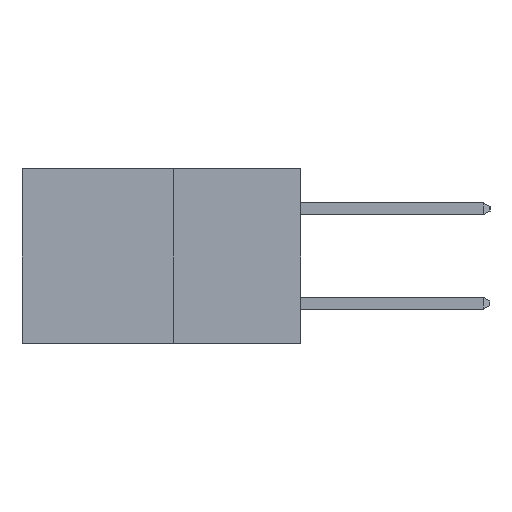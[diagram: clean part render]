
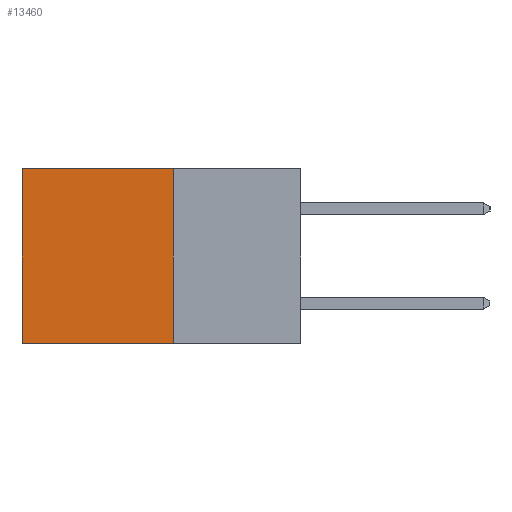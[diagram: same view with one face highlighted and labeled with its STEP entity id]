
A CAD part, left-side view. The second image highlights one B-rep face of the part: STEP entity #13460.
In plain terms, the highlighted planar face has unit normal (-1, 0, 0).
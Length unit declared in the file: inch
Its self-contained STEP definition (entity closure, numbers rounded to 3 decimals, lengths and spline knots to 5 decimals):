
#970 = LINE ( 'NONE', #22688, #26097 ) ;
#2317 = CARTESIAN_POINT ( 'NONE',  ( 0.277, 0.59, -0.37 ) ) ;
#2711 = FACE_OUTER_BOUND ( 'NONE', #18869, .T. ) ;
#3425 = CARTESIAN_POINT ( 'NONE',  ( 0.277, 0.27, -0.37 ) ) ;
#3765 = EDGE_CURVE ( 'NONE', #10732, #7040, #18113, .T. ) ;
#3942 = LINE ( 'NONE', #3425, #16308 ) ;
#4240 = CARTESIAN_POINT ( 'NONE',  ( 0.277, 0.59, -0.37 ) ) ;
#4717 = PLANE ( 'NONE',  #15020 ) ;
#7040 = VERTEX_POINT ( 'NONE', #27132 ) ;
#7058 = VECTOR ( 'NONE', #21379, 39.37008 ) ;
#7215 = DIRECTION ( 'NONE',  ( 1., 0., 0. ) ) ;
#7545 = VERTEX_POINT ( 'NONE', #2317 ) ;
#10732 = VERTEX_POINT ( 'NONE', #27870 ) ;
#10850 = VERTEX_POINT ( 'NONE', #16812 ) ;
#11650 = VECTOR ( 'NONE', #13503, 39.37008 ) ;
#13460 = ADVANCED_FACE ( 'NONE', ( #2711 ), #4717, .F. ) ;
#13503 = DIRECTION ( 'NONE',  ( 0., 1., 0. ) ) ;
#15020 = AXIS2_PLACEMENT_3D ( 'NONE', #21832, #7215, #24189 ) ;
#15191 = CARTESIAN_POINT ( 'NONE',  ( 0.277, 0.27, 0. ) ) ;
#16308 = VECTOR ( 'NONE', #25361, 39.37008 ) ;
#16565 = EDGE_CURVE ( 'NONE', #7040, #7545, #26382, .T. ) ;
#16812 = CARTESIAN_POINT ( 'NONE',  ( 0.277, 0.27, -0.37 ) ) ;
#17372 = ORIENTED_EDGE ( 'NONE', *, *, #3765, .T. ) ;
#18113 = LINE ( 'NONE', #15191, #11650 ) ;
#18438 = ORIENTED_EDGE ( 'NONE', *, *, #16565, .T. ) ;
#18869 = EDGE_LOOP ( 'NONE', ( #18438, #26480, #27967, #17372 ) ) ;
#20419 = DIRECTION ( 'NONE',  ( 0., 1., 0. ) ) ;
#21379 = DIRECTION ( 'NONE',  ( 0., 0., -1. ) ) ;
#21732 = EDGE_CURVE ( 'NONE', #10850, #7545, #970, .T. ) ;
#21832 = CARTESIAN_POINT ( 'NONE',  ( 0.277, 0.27, -0.37 ) ) ;
#22688 = CARTESIAN_POINT ( 'NONE',  ( 0.277, 0.27, -0.37 ) ) ;
#24189 = DIRECTION ( 'NONE',  ( 0., 0., -1. ) ) ;
#25361 = DIRECTION ( 'NONE',  ( 0., 0., -1. ) ) ;
#25578 = EDGE_CURVE ( 'NONE', #10732, #10850, #3942, .T. ) ;
#26097 = VECTOR ( 'NONE', #20419, 39.37008 ) ;
#26382 = LINE ( 'NONE', #4240, #7058 ) ;
#26480 = ORIENTED_EDGE ( 'NONE', *, *, #21732, .F. ) ;
#27132 = CARTESIAN_POINT ( 'NONE',  ( 0.277, 0.59, 0. ) ) ;
#27870 = CARTESIAN_POINT ( 'NONE',  ( 0.277, 0.27, 0. ) ) ;
#27967 = ORIENTED_EDGE ( 'NONE', *, *, #25578, .F. ) ;
